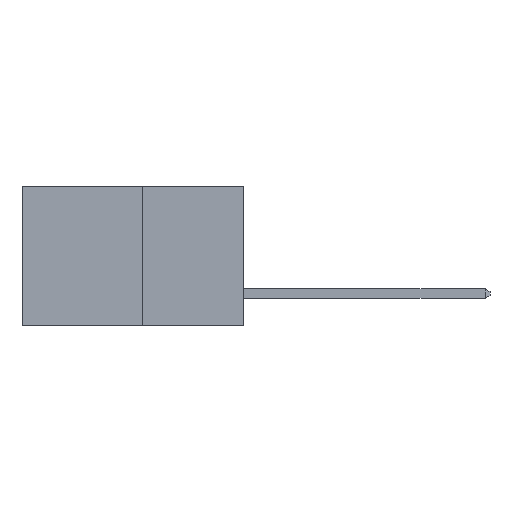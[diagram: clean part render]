
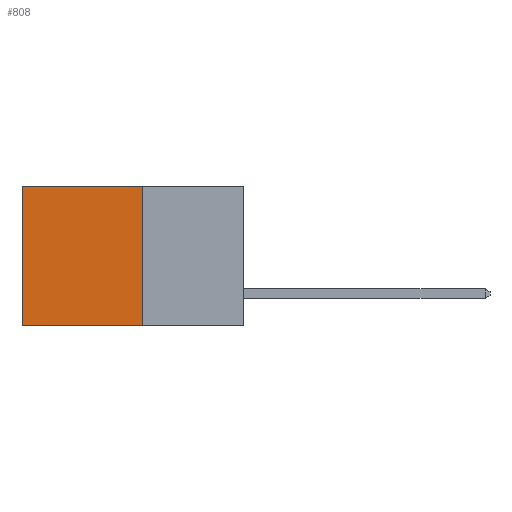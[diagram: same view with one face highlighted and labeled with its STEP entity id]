
A CAD part, left-side view. The second image highlights one B-rep face of the part: STEP entity #808.
In plain terms, the highlighted planar face has unit normal (-1, 0, 0).
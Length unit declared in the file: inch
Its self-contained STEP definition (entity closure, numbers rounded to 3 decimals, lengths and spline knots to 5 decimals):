
#260 = AXIS2_PLACEMENT_3D ( 'NONE', #7926, #5803, #5267 ) ;
#263 = VERTEX_POINT ( 'NONE', #6699 ) ;
#442 = LINE ( 'NONE', #4830, #2512 ) ;
#808 = ADVANCED_FACE ( 'NONE', ( #6641 ), #8324, .F. ) ;
#903 = EDGE_CURVE ( 'NONE', #1652, #3108, #2664, .T. ) ;
#1534 = VERTEX_POINT ( 'NONE', #6970 ) ;
#1652 = VERTEX_POINT ( 'NONE', #5653 ) ;
#1723 = EDGE_CURVE ( 'NONE', #1534, #3108, #6360, .T. ) ;
#2512 = VECTOR ( 'NONE', #7890, 39.37008 ) ;
#2664 = LINE ( 'NONE', #4551, #5882 ) ;
#2705 = VECTOR ( 'NONE', #3612, 39.37008 ) ;
#2832 = EDGE_CURVE ( 'NONE', #263, #1652, #442, .T. ) ;
#3108 = VERTEX_POINT ( 'NONE', #3965 ) ;
#3228 = EDGE_LOOP ( 'NONE', ( #6820, #4458, #4903, #6265 ) ) ;
#3612 = DIRECTION ( 'NONE',  ( 0., 1., 0. ) ) ;
#3719 = EDGE_CURVE ( 'NONE', #263, #1534, #7523, .T. ) ;
#3935 = DIRECTION ( 'NONE',  ( 0., 1., 0. ) ) ;
#3965 = CARTESIAN_POINT ( 'NONE',  ( 0.277, 0.59, -0.37 ) ) ;
#4458 = ORIENTED_EDGE ( 'NONE', *, *, #903, .F. ) ;
#4551 = CARTESIAN_POINT ( 'NONE',  ( 0.277, 0.27, -0.37 ) ) ;
#4706 = VECTOR ( 'NONE', #6541, 39.37008 ) ;
#4830 = CARTESIAN_POINT ( 'NONE',  ( 0.277, 0.27, -0.37 ) ) ;
#4903 = ORIENTED_EDGE ( 'NONE', *, *, #2832, .F. ) ;
#5267 = DIRECTION ( 'NONE',  ( 0., 0., -1. ) ) ;
#5306 = CARTESIAN_POINT ( 'NONE',  ( 0.277, 0.27, 0. ) ) ;
#5653 = CARTESIAN_POINT ( 'NONE',  ( 0.277, 0.27, -0.37 ) ) ;
#5803 = DIRECTION ( 'NONE',  ( 1., 0., 0. ) ) ;
#5882 = VECTOR ( 'NONE', #3935, 39.37008 ) ;
#6265 = ORIENTED_EDGE ( 'NONE', *, *, #3719, .T. ) ;
#6360 = LINE ( 'NONE', #7718, #4706 ) ;
#6541 = DIRECTION ( 'NONE',  ( 0., 0., -1. ) ) ;
#6641 = FACE_OUTER_BOUND ( 'NONE', #3228, .T. ) ;
#6699 = CARTESIAN_POINT ( 'NONE',  ( 0.277, 0.27, 0. ) ) ;
#6820 = ORIENTED_EDGE ( 'NONE', *, *, #1723, .T. ) ;
#6970 = CARTESIAN_POINT ( 'NONE',  ( 0.277, 0.59, 0. ) ) ;
#7523 = LINE ( 'NONE', #5306, #2705 ) ;
#7718 = CARTESIAN_POINT ( 'NONE',  ( 0.277, 0.59, -0.37 ) ) ;
#7890 = DIRECTION ( 'NONE',  ( 0., 0., -1. ) ) ;
#7926 = CARTESIAN_POINT ( 'NONE',  ( 0.277, 0.27, -0.37 ) ) ;
#8324 = PLANE ( 'NONE',  #260 ) ;
